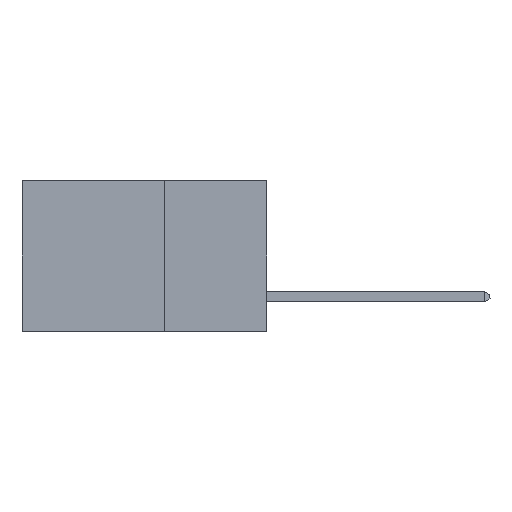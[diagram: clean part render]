
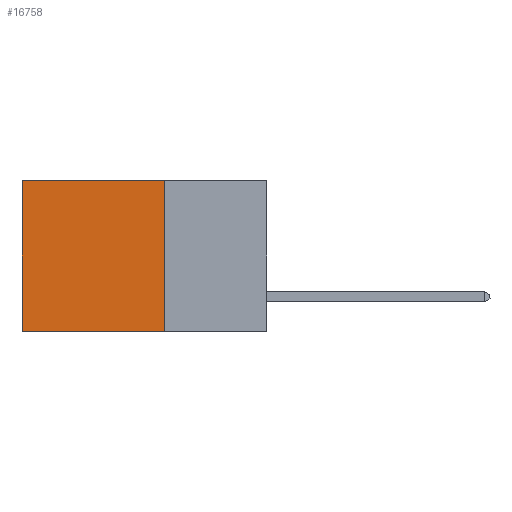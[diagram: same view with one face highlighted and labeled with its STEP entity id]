
A CAD part, left-side view. The second image highlights one B-rep face of the part: STEP entity #16758.
In plain terms, the highlighted planar face has unit normal (-1, 0, 0).
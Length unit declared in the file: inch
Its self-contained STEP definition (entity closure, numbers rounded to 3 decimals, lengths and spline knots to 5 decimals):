
#90 = EDGE_CURVE ( 'NONE', #3622, #4894, #1070, .T. ) ;
#1070 = LINE ( 'NONE', #16189, #7916 ) ;
#1187 = FACE_OUTER_BOUND ( 'NONE', #8539, .T. ) ;
#1598 = DIRECTION ( 'NONE',  ( 0., 1., 0. ) ) ;
#1603 = LINE ( 'NONE', #3050, #12049 ) ;
#2172 = EDGE_CURVE ( 'NONE', #14089, #7461, #6083, .T. ) ;
#2469 = VECTOR ( 'NONE', #9540, 39.37008 ) ;
#3050 = CARTESIAN_POINT ( 'NONE',  ( 0.2875, 0.25, -0.37 ) ) ;
#3622 = VERTEX_POINT ( 'NONE', #9372 ) ;
#3780 = ORIENTED_EDGE ( 'NONE', *, *, #2172, .F. ) ;
#4420 = ORIENTED_EDGE ( 'NONE', *, *, #16600, .T. ) ;
#4832 = CARTESIAN_POINT ( 'NONE',  ( 0.2875, 0.25, 0. ) ) ;
#4894 = VERTEX_POINT ( 'NONE', #9043 ) ;
#5463 = CARTESIAN_POINT ( 'NONE',  ( 0.2875, 0.25, 0. ) ) ;
#6083 = LINE ( 'NONE', #10111, #2469 ) ;
#6191 = DIRECTION ( 'NONE',  ( 0., 0., -1. ) ) ;
#6451 = AXIS2_PLACEMENT_3D ( 'NONE', #4832, #14188, #6191 ) ;
#6727 = VECTOR ( 'NONE', #12563, 39.37008 ) ;
#7461 = VERTEX_POINT ( 'NONE', #8999 ) ;
#7916 = VECTOR ( 'NONE', #11840, 39.37008 ) ;
#8539 = EDGE_LOOP ( 'NONE', ( #15648, #15444, #3780, #4420 ) ) ;
#8999 = CARTESIAN_POINT ( 'NONE',  ( 0.2875, 0.25, -0.37 ) ) ;
#9043 = CARTESIAN_POINT ( 'NONE',  ( 0.2875, 0.6, -0.37 ) ) ;
#9372 = CARTESIAN_POINT ( 'NONE',  ( 0.2875, 0.6, 0. ) ) ;
#9540 = DIRECTION ( 'NONE',  ( 0., 0., -1. ) ) ;
#10111 = CARTESIAN_POINT ( 'NONE',  ( 0.2875, 0.25, 0. ) ) ;
#10338 = LINE ( 'NONE', #11258, #6727 ) ;
#10802 = EDGE_CURVE ( 'NONE', #7461, #4894, #1603, .T. ) ;
#11258 = CARTESIAN_POINT ( 'NONE',  ( 0.2875, 0.25, 0. ) ) ;
#11611 = PLANE ( 'NONE',  #6451 ) ;
#11840 = DIRECTION ( 'NONE',  ( 0., 0., -1. ) ) ;
#12049 = VECTOR ( 'NONE', #1598, 39.37008 ) ;
#12563 = DIRECTION ( 'NONE',  ( 0., 1., 0. ) ) ;
#14089 = VERTEX_POINT ( 'NONE', #5463 ) ;
#14188 = DIRECTION ( 'NONE',  ( 1., 0., 0. ) ) ;
#15444 = ORIENTED_EDGE ( 'NONE', *, *, #10802, .F. ) ;
#15648 = ORIENTED_EDGE ( 'NONE', *, *, #90, .T. ) ;
#16189 = CARTESIAN_POINT ( 'NONE',  ( 0.2875, 0.6, 0. ) ) ;
#16600 = EDGE_CURVE ( 'NONE', #14089, #3622, #10338, .T. ) ;
#16758 = ADVANCED_FACE ( 'NONE', ( #1187 ), #11611, .F. ) ;
